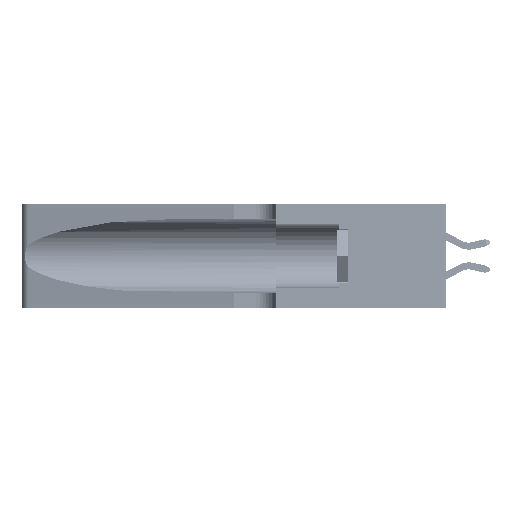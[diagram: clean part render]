
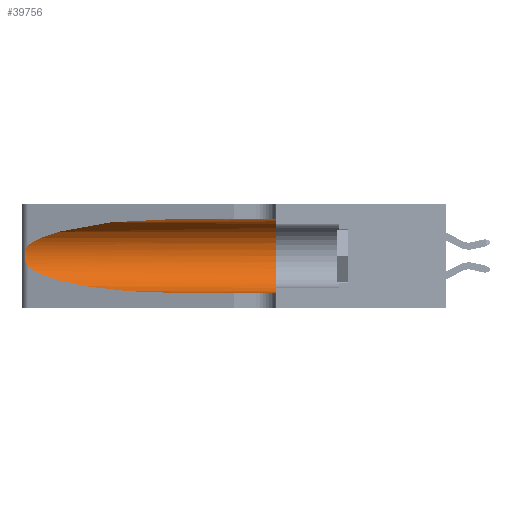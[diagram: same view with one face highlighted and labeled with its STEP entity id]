
A CAD part, left-side view. The second image highlights one B-rep face of the part: STEP entity #39756.
In plain terms, the highlighted cylindrical face has radius 3.308 mm (diameter 6.617 mm), a partial arc.
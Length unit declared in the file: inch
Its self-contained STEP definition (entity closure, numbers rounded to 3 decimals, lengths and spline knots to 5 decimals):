
#1435 = CARTESIAN_POINT ( 'NONE',  ( 0.1305, 0.72297, 0.05475 ) ) ;
#1689 = VECTOR ( 'NONE', #26079, 39.37008 ) ;
#1772 = CARTESIAN_POINT ( 'NONE',  ( 0.1305, 1.61858, 0.31525 ) ) ;
#2454 = EDGE_CURVE ( 'NONE', #7965, #28977, #5028, .T. ) ;
#3459 = CARTESIAN_POINT ( 'NONE',  ( 0.25487, 1.22718, 0.14631 ) ) ;
#4228 = CARTESIAN_POINT ( 'NONE',  ( 0.25787, 1.23484, 0.2124 ) ) ;
#5028 =( BOUNDED_CURVE ( )  B_SPLINE_CURVE ( 3, ( #30185, #34243, #38383, #42472 ),
 .UNSPECIFIED., .F., .F. ) 
 B_SPLINE_CURVE_WITH_KNOTS ( ( 4, 4 ),
 ( 3.44316, 4.71239 ),
 .UNSPECIFIED. ) 
 CURVE ( )  GEOMETRIC_REPRESENTATION_ITEM ( )  RATIONAL_B_SPLINE_CURVE ( ( 1., 0.87, 0.87, 1. ) ) 
 REPRESENTATION_ITEM ( '' )  );
#5086 = VERTEX_POINT ( 'NONE', #50863 ) ;
#7399 = EDGE_CURVE ( 'NONE', #5086, #7965, #34290, .T. ) ;
#7965 = VERTEX_POINT ( 'NONE', #3459 ) ;
#8377 = CARTESIAN_POINT ( 'NONE',  ( 0.26018, 1.23835, 0.19895 ) ) ;
#8660 = DIRECTION ( 'NONE',  ( 0., -1., 0. ) ) ;
#10294 = CARTESIAN_POINT ( 'NONE',  ( 0.1305, 1.61858, 0.05475 ) ) ;
#10333 = CARTESIAN_POINT ( 'NONE',  ( 0.1305, 0.35, 0.31525 ) ) ;
#11767 = EDGE_CURVE ( 'NONE', #44588, #12493, #43858, .T. ) ;
#11995 = FACE_OUTER_BOUND ( 'NONE', #31623, .T. ) ;
#12472 = CARTESIAN_POINT ( 'NONE',  ( 0.26075, 1.23896, 0.178 ) ) ;
#12493 = VERTEX_POINT ( 'NONE', #10333 ) ;
#12761 = DIRECTION ( 'NONE',  ( 0., 0., -1. ) ) ;
#12763 = ORIENTED_EDGE ( 'NONE', *, *, #7399, .T. ) ;
#13100 = CARTESIAN_POINT ( 'NONE',  ( 0.1305, 0.35, 0.185 ) ) ;
#13164 = CARTESIAN_POINT ( 'NONE',  ( 0.1305, 0.72297, 0.31525 ) ) ;
#14394 = DIRECTION ( 'NONE',  ( 0., -1., 0. ) ) ;
#14550 = LINE ( 'NONE', #10294, #45813 ) ;
#16589 = CARTESIAN_POINT ( 'NONE',  ( 0.25856, 1.23593, 0.16098 ) ) ;
#17221 = DIRECTION ( 'NONE',  ( 0., 0., 1. ) ) ;
#17447 = ORIENTED_EDGE ( 'NONE', *, *, #2454, .T. ) ;
#18308 = ORIENTED_EDGE ( 'NONE', *, *, #26007, .T. ) ;
#20284 = CYLINDRICAL_SURFACE ( 'NONE', #48133, 0.13025 ) ;
#20684 = CARTESIAN_POINT ( 'NONE',  ( 0.25639, 1.23186, 0.15144 ) ) ;
#20800 = ORIENTED_EDGE ( 'NONE', *, *, #48457, .F. ) ;
#21367 = CARTESIAN_POINT ( 'NONE',  ( 0.2373, 1.15595, 0.28018 ) ) ;
#24768 = CARTESIAN_POINT ( 'NONE',  ( 0.25487, 1.22718, 0.14631 ) ) ;
#25289 = CARTESIAN_POINT ( 'NONE',  ( 0.18966, 0.96281, 0.31525 ) ) ;
#26007 = EDGE_CURVE ( 'NONE', #28977, #40816, #14550, .T. ) ;
#26079 = DIRECTION ( 'NONE',  ( 0., -1., 0. ) ) ;
#26732 = ORIENTED_EDGE ( 'NONE', *, *, #51549, .T. ) ;
#28689 = CARTESIAN_POINT ( 'NONE',  ( 0.25639, 1.23184, 0.21858 ) ) ;
#28977 = VERTEX_POINT ( 'NONE', #1435 ) ;
#30185 = CARTESIAN_POINT ( 'NONE',  ( 0.25487, 1.22718, 0.14631 ) ) ;
#31623 = EDGE_LOOP ( 'NONE', ( #26732, #12763, #17447, #18308, #20800, #32271 ) ) ;
#32271 = ORIENTED_EDGE ( 'NONE', *, *, #11767, .F. ) ;
#32762 = CARTESIAN_POINT ( 'NONE',  ( 0.25854, 1.2359, 0.20912 ) ) ;
#34243 = CARTESIAN_POINT ( 'NONE',  ( 0.2373, 1.15595, 0.08982 ) ) ;
#34290 = B_SPLINE_CURVE_WITH_KNOTS ( 'NONE', 3,
 ( #40822, #49042, #28689, #4228, #32762, #8377, #36876, #12472, #40989, #16589, #45104, #20684, #49237, #24768 ),
 .UNSPECIFIED., .F., .F.,
 ( 4, 2, 2, 2, 2, 2, 4 ),
 ( 0., 0.00027, 0.00053, 0.00107, 0.0016, 0.00187, 0.00214 ),
 .UNSPECIFIED. ) ;
#36876 = CARTESIAN_POINT ( 'NONE',  ( 0.26075, 1.23896, 0.19203 ) ) ;
#38383 = CARTESIAN_POINT ( 'NONE',  ( 0.18966, 0.96281, 0.05475 ) ) ;
#39756 = ADVANCED_FACE ( 'NONE', ( #11995 ), #20284, .F. ) ;
#40362 = CIRCLE ( 'NONE', #44407, 0.13025 ) ;
#40816 = VERTEX_POINT ( 'NONE', #51767 ) ;
#40822 = CARTESIAN_POINT ( 'NONE',  ( 0.25487, 1.22718, 0.22369 ) ) ;
#40989 = CARTESIAN_POINT ( 'NONE',  ( 0.26017, 1.23833, 0.17102 ) ) ;
#41620 = DIRECTION ( 'NONE',  ( 0., 1., 0. ) ) ;
#42472 = CARTESIAN_POINT ( 'NONE',  ( 0.1305, 0.72297, 0.05475 ) ) ;
#43858 = LINE ( 'NONE', #1772, #1689 ) ;
#44407 = AXIS2_PLACEMENT_3D ( 'NONE', #13100, #41620, #17221 ) ;
#44588 = VERTEX_POINT ( 'NONE', #48405 ) ;
#45104 = CARTESIAN_POINT ( 'NONE',  ( 0.25789, 1.23486, 0.15765 ) ) ;
#45813 = VECTOR ( 'NONE', #14394, 39.37008 ) ;
#48133 = AXIS2_PLACEMENT_3D ( 'NONE', #49346, #8660, #12761 ) ;
#48405 = CARTESIAN_POINT ( 'NONE',  ( 0.1305, 0.72297, 0.31525 ) ) ;
#48457 = EDGE_CURVE ( 'NONE', #12493, #40816, #40362, .T. ) ;
#49042 = CARTESIAN_POINT ( 'NONE',  ( 0.25555, 1.22994, 0.2215 ) ) ;
#49237 = CARTESIAN_POINT ( 'NONE',  ( 0.25555, 1.22993, 0.14849 ) ) ;
#49346 = CARTESIAN_POINT ( 'NONE',  ( 0.1305, 1.61858, 0.185 ) ) ;
#49926 = CARTESIAN_POINT ( 'NONE',  ( 0.25487, 1.22718, 0.22369 ) ) ;
#50863 = CARTESIAN_POINT ( 'NONE',  ( 0.25487, 1.22718, 0.22369 ) ) ;
#51549 = EDGE_CURVE ( 'NONE', #44588, #5086, #52620, .T. ) ;
#51767 = CARTESIAN_POINT ( 'NONE',  ( 0.1305, 0.35, 0.05475 ) ) ;
#52620 =( BOUNDED_CURVE ( )  B_SPLINE_CURVE ( 3, ( #13164, #25289, #21367, #49926 ),
 .UNSPECIFIED., .F., .T. ) 
 B_SPLINE_CURVE_WITH_KNOTS ( ( 4, 4 ),
 ( 1.5708, 2.84003 ),
 .UNSPECIFIED. ) 
 CURVE ( )  GEOMETRIC_REPRESENTATION_ITEM ( )  RATIONAL_B_SPLINE_CURVE ( ( 1., 0.87, 0.87, 1. ) ) 
 REPRESENTATION_ITEM ( '' )  );
